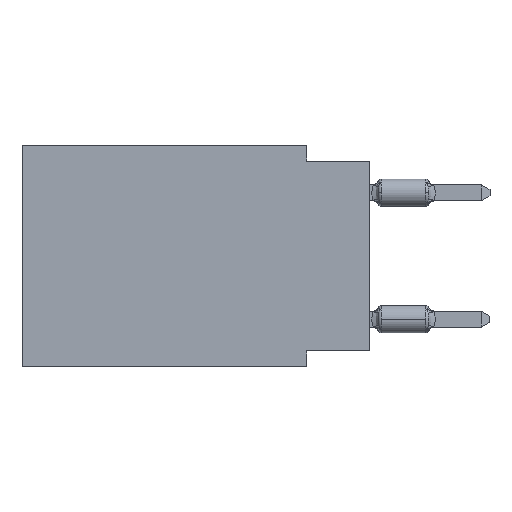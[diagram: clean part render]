
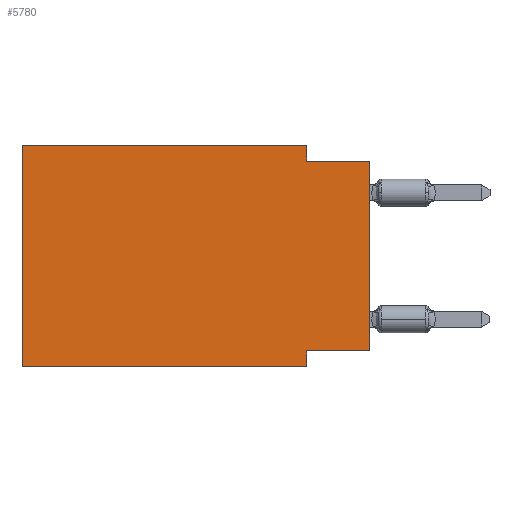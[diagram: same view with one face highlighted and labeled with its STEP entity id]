
A CAD part, left-side view. The second image highlights one B-rep face of the part: STEP entity #5780.
In plain terms, the highlighted planar face has unit normal (-1, 0, 0).
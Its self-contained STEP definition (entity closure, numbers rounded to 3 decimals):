
#123 = LINE ( 'NONE', #8633, #3302 ) ;
#265 = LINE ( 'NONE', #7532, #6994 ) ;
#267 = LINE ( 'NONE', #5372, #4412 ) ;
#401 = ORIENTED_EDGE ( 'NONE', *, *, #6616, .F. ) ;
#481 = PLANE ( 'NONE',  #485 ) ;
#485 = AXIS2_PLACEMENT_3D ( 'NONE', #7878, #614, #11085 ) ;
#584 = ORIENTED_EDGE ( 'NONE', *, *, #12180, .T. ) ;
#614 = DIRECTION ( 'NONE',  ( 1., 0., 0. ) ) ;
#634 = CARTESIAN_POINT ( 'NONE',  ( 0., 13.97, 0. ) ) ;
#922 = ORIENTED_EDGE ( 'NONE', *, *, #9854, .F. ) ;
#1074 = DIRECTION ( 'NONE',  ( 0., 0., 1. ) ) ;
#1253 = CARTESIAN_POINT ( 'NONE',  ( 0., 0., -8.255 ) ) ;
#1303 = VERTEX_POINT ( 'NONE', #4699 ) ;
#1523 = FACE_OUTER_BOUND ( 'NONE', #3254, .T. ) ;
#1671 = LINE ( 'NONE', #634, #2757 ) ;
#1676 = DIRECTION ( 'NONE',  ( 0., -1., 0. ) ) ;
#1850 = EDGE_CURVE ( 'NONE', #6621, #10611, #13689, .T. ) ;
#2112 = CARTESIAN_POINT ( 'NONE',  ( 0., 0., 0. ) ) ;
#2286 = LINE ( 'NONE', #1253, #5436 ) ;
#2395 = CARTESIAN_POINT ( 'NONE',  ( 0., 0., -8.255 ) ) ;
#2446 = ORIENTED_EDGE ( 'NONE', *, *, #10588, .F. ) ;
#2451 = VERTEX_POINT ( 'NONE', #4358 ) ;
#2452 = CARTESIAN_POINT ( 'NONE',  ( 0., 2.54, -0.635 ) ) ;
#2757 = VECTOR ( 'NONE', #6021, 1000. ) ;
#3254 = EDGE_LOOP ( 'NONE', ( #8138, #3811, #9835, #401, #922, #584, #2446, #10739 ) ) ;
#3302 = VECTOR ( 'NONE', #12892, 1000. ) ;
#3346 = VERTEX_POINT ( 'NONE', #3620 ) ;
#3355 = LINE ( 'NONE', #2112, #11010 ) ;
#3575 = DIRECTION ( 'NONE',  ( 0., -1., 0. ) ) ;
#3620 = CARTESIAN_POINT ( 'NONE',  ( 0., 13.97, 0. ) ) ;
#3811 = ORIENTED_EDGE ( 'NONE', *, *, #1850, .F. ) ;
#4111 = DIRECTION ( 'NONE',  ( 0., 1., 0. ) ) ;
#4358 = CARTESIAN_POINT ( 'NONE',  ( 0., 2.54, -8.89 ) ) ;
#4412 = VECTOR ( 'NONE', #8572, 1000. ) ;
#4699 = CARTESIAN_POINT ( 'NONE',  ( 0., 13.97, -8.89 ) ) ;
#5372 = CARTESIAN_POINT ( 'NONE',  ( 0., 2.54, -8.89 ) ) ;
#5436 = VECTOR ( 'NONE', #4111, 1000. ) ;
#5780 = ADVANCED_FACE ( 'NONE', ( #1523 ), #481, .F. ) ;
#6021 = DIRECTION ( 'NONE',  ( 0., 0., 1. ) ) ;
#6555 = CARTESIAN_POINT ( 'NONE',  ( 0., 0., -0.635 ) ) ;
#6616 = EDGE_CURVE ( 'NONE', #3346, #7566, #7642, .T. ) ;
#6621 = VERTEX_POINT ( 'NONE', #2452 ) ;
#6994 = VECTOR ( 'NONE', #10593, 1000. ) ;
#7132 = VERTEX_POINT ( 'NONE', #9841 ) ;
#7405 = EDGE_CURVE ( 'NONE', #12100, #7132, #2286, .T. ) ;
#7532 = CARTESIAN_POINT ( 'NONE',  ( 0., 2.54, 0. ) ) ;
#7566 = VERTEX_POINT ( 'NONE', #11218 ) ;
#7642 = LINE ( 'NONE', #10843, #12760 ) ;
#7878 = CARTESIAN_POINT ( 'NONE',  ( 0., 13.97, 0. ) ) ;
#8097 = EDGE_CURVE ( 'NONE', #12100, #10611, #3355, .T. ) ;
#8138 = ORIENTED_EDGE ( 'NONE', *, *, #8097, .T. ) ;
#8473 = VECTOR ( 'NONE', #1676, 1000. ) ;
#8572 = DIRECTION ( 'NONE',  ( 0., 0., -1. ) ) ;
#8633 = CARTESIAN_POINT ( 'NONE',  ( 0., 13.97, -8.89 ) ) ;
#9289 = EDGE_CURVE ( 'NONE', #7566, #6621, #265, .T. ) ;
#9835 = ORIENTED_EDGE ( 'NONE', *, *, #9289, .F. ) ;
#9841 = CARTESIAN_POINT ( 'NONE',  ( 0., 2.54, -8.255 ) ) ;
#9854 = EDGE_CURVE ( 'NONE', #1303, #3346, #1671, .T. ) ;
#10588 = EDGE_CURVE ( 'NONE', #7132, #2451, #267, .T. ) ;
#10593 = DIRECTION ( 'NONE',  ( 0., 0., -1. ) ) ;
#10611 = VERTEX_POINT ( 'NONE', #6555 ) ;
#10739 = ORIENTED_EDGE ( 'NONE', *, *, #7405, .F. ) ;
#10843 = CARTESIAN_POINT ( 'NONE',  ( 0., 13.97, 0. ) ) ;
#11010 = VECTOR ( 'NONE', #1074, 1000. ) ;
#11085 = DIRECTION ( 'NONE',  ( 0., 0., -1. ) ) ;
#11218 = CARTESIAN_POINT ( 'NONE',  ( 0., 2.54, 0. ) ) ;
#12100 = VERTEX_POINT ( 'NONE', #2395 ) ;
#12180 = EDGE_CURVE ( 'NONE', #1303, #2451, #123, .T. ) ;
#12760 = VECTOR ( 'NONE', #3575, 1000. ) ;
#12892 = DIRECTION ( 'NONE',  ( 0., -1., 0. ) ) ;
#13621 = CARTESIAN_POINT ( 'NONE',  ( 0., 0., -0.635 ) ) ;
#13689 = LINE ( 'NONE', #13621, #8473 ) ;
